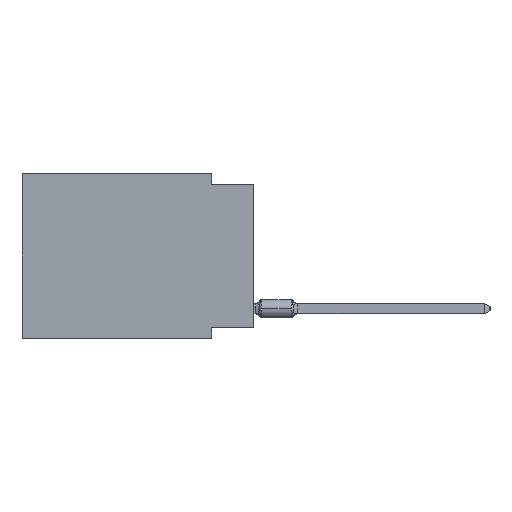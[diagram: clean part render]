
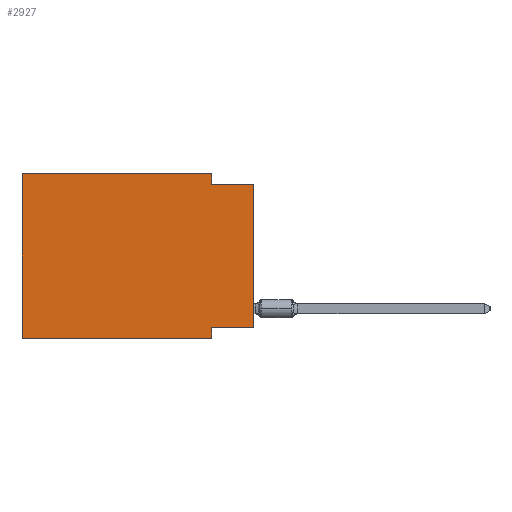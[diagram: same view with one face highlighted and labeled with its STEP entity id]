
A CAD part, left-side view. The second image highlights one B-rep face of the part: STEP entity #2927.
In plain terms, the highlighted planar face has unit normal (-1, 0, 0).
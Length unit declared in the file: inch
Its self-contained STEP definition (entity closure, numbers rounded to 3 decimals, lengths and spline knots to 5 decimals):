
#1394 = CARTESIAN_POINT ( 'NONE',  ( 0., 0.1, 0. ) ) ;
#1683 = VECTOR ( 'NONE', #8340, 39.37008 ) ;
#2876 = EDGE_CURVE ( 'NONE', #4085, #13055, #26936, .T. ) ;
#2927 = ADVANCED_FACE ( 'NONE', ( #3413 ), #13594, .F. ) ;
#3110 = ORIENTED_EDGE ( 'NONE', *, *, #6901, .T. ) ;
#3413 = FACE_OUTER_BOUND ( 'NONE', #22424, .T. ) ;
#3417 = VECTOR ( 'NONE', #7350, 39.37008 ) ;
#4085 = VERTEX_POINT ( 'NONE', #17970 ) ;
#4777 = ORIENTED_EDGE ( 'NONE', *, *, #19458, .T. ) ;
#5637 = CARTESIAN_POINT ( 'NONE',  ( 0., 0.1, -0.025 ) ) ;
#5677 = ORIENTED_EDGE ( 'NONE', *, *, #24304, .F. ) ;
#5714 = CARTESIAN_POINT ( 'NONE',  ( 0., 0.55, 0. ) ) ;
#5943 = VERTEX_POINT ( 'NONE', #1394 ) ;
#6590 = CARTESIAN_POINT ( 'NONE',  ( 0., 0., -0.025 ) ) ;
#6901 = EDGE_CURVE ( 'NONE', #30888, #11825, #18503, .T. ) ;
#7293 = CARTESIAN_POINT ( 'NONE',  ( 0., 0.55, 0. ) ) ;
#7350 = DIRECTION ( 'NONE',  ( 0., 0., -1. ) ) ;
#7667 = ORIENTED_EDGE ( 'NONE', *, *, #13271, .F. ) ;
#8340 = DIRECTION ( 'NONE',  ( 0., 0., 1. ) ) ;
#9191 = DIRECTION ( 'NONE',  ( 0., -1., 0. ) ) ;
#10460 = VECTOR ( 'NONE', #11680, 39.37008 ) ;
#10936 = EDGE_CURVE ( 'NONE', #23736, #16980, #33670, .T. ) ;
#11012 = DIRECTION ( 'NONE',  ( 0., -1., 0. ) ) ;
#11371 = VECTOR ( 'NONE', #9191, 39.37008 ) ;
#11537 = VECTOR ( 'NONE', #16206, 39.37008 ) ;
#11680 = DIRECTION ( 'NONE',  ( 0., -1., 0. ) ) ;
#11825 = VERTEX_POINT ( 'NONE', #6590 ) ;
#13055 = VERTEX_POINT ( 'NONE', #7293 ) ;
#13271 = EDGE_CURVE ( 'NONE', #13055, #5943, #14453, .T. ) ;
#13328 = LINE ( 'NONE', #18778, #18371 ) ;
#13594 = PLANE ( 'NONE',  #14578 ) ;
#14091 = LINE ( 'NONE', #29542, #11537 ) ;
#14453 = LINE ( 'NONE', #27100, #11371 ) ;
#14578 = AXIS2_PLACEMENT_3D ( 'NONE', #29742, #27460, #29567 ) ;
#15650 = VECTOR ( 'NONE', #28851, 39.37008 ) ;
#16037 = VECTOR ( 'NONE', #11012, 39.37008 ) ;
#16206 = DIRECTION ( 'NONE',  ( 0., 1., 0. ) ) ;
#16980 = VERTEX_POINT ( 'NONE', #25740 ) ;
#17697 = CARTESIAN_POINT ( 'NONE',  ( 0., 0.1, -0.39 ) ) ;
#17970 = CARTESIAN_POINT ( 'NONE',  ( 0., 0.55, -0.39 ) ) ;
#18371 = VECTOR ( 'NONE', #29483, 39.37008 ) ;
#18414 = CARTESIAN_POINT ( 'NONE',  ( 0., 0., -0.025 ) ) ;
#18503 = LINE ( 'NONE', #26225, #15650 ) ;
#18778 = CARTESIAN_POINT ( 'NONE',  ( 0., 0.1, 0. ) ) ;
#19458 = EDGE_CURVE ( 'NONE', #4085, #16980, #29944, .T. ) ;
#20240 = EDGE_CURVE ( 'NONE', #5943, #22867, #13328, .T. ) ;
#22424 = EDGE_LOOP ( 'NONE', ( #3110, #5677, #25470, #7667, #22444, #4777, #34543, #28763 ) ) ;
#22444 = ORIENTED_EDGE ( 'NONE', *, *, #2876, .F. ) ;
#22867 = VERTEX_POINT ( 'NONE', #5637 ) ;
#23593 = EDGE_CURVE ( 'NONE', #30888, #23736, #14091, .T. ) ;
#23736 = VERTEX_POINT ( 'NONE', #27607 ) ;
#24304 = EDGE_CURVE ( 'NONE', #22867, #11825, #27005, .T. ) ;
#24517 = CARTESIAN_POINT ( 'NONE',  ( 0., 0.55, -0.39 ) ) ;
#25470 = ORIENTED_EDGE ( 'NONE', *, *, #20240, .F. ) ;
#25740 = CARTESIAN_POINT ( 'NONE',  ( 0., 0.1, -0.39 ) ) ;
#26225 = CARTESIAN_POINT ( 'NONE',  ( 0., 0., 0. ) ) ;
#26936 = LINE ( 'NONE', #5714, #1683 ) ;
#27005 = LINE ( 'NONE', #18414, #16037 ) ;
#27100 = CARTESIAN_POINT ( 'NONE',  ( 0., 0.55, 0. ) ) ;
#27460 = DIRECTION ( 'NONE',  ( 1., 0., 0. ) ) ;
#27607 = CARTESIAN_POINT ( 'NONE',  ( 0., 0.1, -0.365 ) ) ;
#28763 = ORIENTED_EDGE ( 'NONE', *, *, #23593, .F. ) ;
#28851 = DIRECTION ( 'NONE',  ( 0., 0., 1. ) ) ;
#29483 = DIRECTION ( 'NONE',  ( 0., 0., -1. ) ) ;
#29542 = CARTESIAN_POINT ( 'NONE',  ( 0., 0., -0.365 ) ) ;
#29567 = DIRECTION ( 'NONE',  ( 0., 0., -1. ) ) ;
#29742 = CARTESIAN_POINT ( 'NONE',  ( 0., 0.55, 0. ) ) ;
#29944 = LINE ( 'NONE', #24517, #10460 ) ;
#30464 = CARTESIAN_POINT ( 'NONE',  ( 0., 0., -0.365 ) ) ;
#30888 = VERTEX_POINT ( 'NONE', #30464 ) ;
#33670 = LINE ( 'NONE', #17697, #3417 ) ;
#34543 = ORIENTED_EDGE ( 'NONE', *, *, #10936, .F. ) ;
